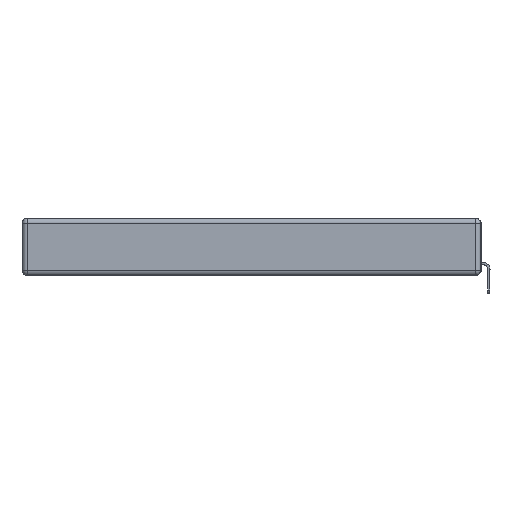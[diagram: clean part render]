
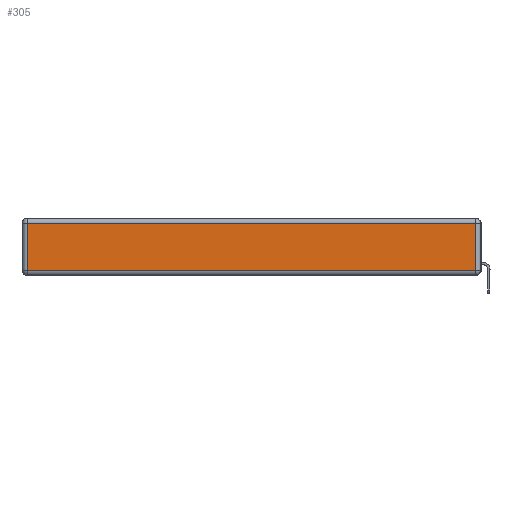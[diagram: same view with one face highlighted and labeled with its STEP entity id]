
A CAD part, left-side view. The second image highlights one B-rep face of the part: STEP entity #305.
In plain terms, the highlighted planar face has unit normal (-1, 0, 0).
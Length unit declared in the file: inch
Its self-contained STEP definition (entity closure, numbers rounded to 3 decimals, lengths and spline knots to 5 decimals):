
#305 = ADVANCED_FACE ( 'NONE', ( #16633 ), #11676, .T. ) ;
#1198 = DIRECTION ( 'NONE',  ( 0., 0., 1. ) ) ;
#1295 = ORIENTED_EDGE ( 'NONE', *, *, #4385, .T. ) ;
#2256 = VERTEX_POINT ( 'NONE', #5201 ) ;
#2484 = ORIENTED_EDGE ( 'NONE', *, *, #16895, .T. ) ;
#2936 = CARTESIAN_POINT ( 'NONE',  ( 0., 0., -0.343 ) ) ;
#4385 = EDGE_CURVE ( 'NONE', #16266, #7479, #18119, .T. ) ;
#4437 = CARTESIAN_POINT ( 'NONE',  ( 0., 2.75, -0.03 ) ) ;
#4552 = LINE ( 'NONE', #4437, #10740 ) ;
#5201 = CARTESIAN_POINT ( 'NONE',  ( 0., 0.03, -0.313 ) ) ;
#6380 = AXIS2_PLACEMENT_3D ( 'NONE', #2936, #9952, #1198 ) ;
#7362 = VERTEX_POINT ( 'NONE', #20991 ) ;
#7479 = VERTEX_POINT ( 'NONE', #11413 ) ;
#8921 = CARTESIAN_POINT ( 'NONE',  ( 0., 2.72, -0.343 ) ) ;
#9952 = DIRECTION ( 'NONE',  ( -1., 0., 0. ) ) ;
#10740 = VECTOR ( 'NONE', #14931, 39.37008 ) ;
#11413 = CARTESIAN_POINT ( 'NONE',  ( 0., 2.72, -0.313 ) ) ;
#11473 = ORIENTED_EDGE ( 'NONE', *, *, #18775, .T. ) ;
#11676 = PLANE ( 'NONE',  #6380 ) ;
#12119 = VECTOR ( 'NONE', #18735, 39.37008 ) ;
#12217 = VECTOR ( 'NONE', #22019, 39.37008 ) ;
#12867 = EDGE_LOOP ( 'NONE', ( #2484, #16663, #11473, #1295 ) ) ;
#13571 = CARTESIAN_POINT ( 'NONE',  ( 0., 0., -0.313 ) ) ;
#14931 = DIRECTION ( 'NONE',  ( 0., 1., 0. ) ) ;
#15064 = LINE ( 'NONE', #13571, #12119 ) ;
#16266 = VERTEX_POINT ( 'NONE', #21402 ) ;
#16633 = FACE_OUTER_BOUND ( 'NONE', #12867, .T. ) ;
#16663 = ORIENTED_EDGE ( 'NONE', *, *, #19182, .T. ) ;
#16895 = EDGE_CURVE ( 'NONE', #7479, #2256, #15064, .T. ) ;
#17077 = CARTESIAN_POINT ( 'NONE',  ( 0., 0.03, -0.343 ) ) ;
#18119 = LINE ( 'NONE', #8921, #21364 ) ;
#18735 = DIRECTION ( 'NONE',  ( 0., -1., 0. ) ) ;
#18775 = EDGE_CURVE ( 'NONE', #7362, #16266, #4552, .T. ) ;
#18794 = LINE ( 'NONE', #17077, #12217 ) ;
#19182 = EDGE_CURVE ( 'NONE', #2256, #7362, #18794, .T. ) ;
#19500 = DIRECTION ( 'NONE',  ( 0., 0., -1. ) ) ;
#20991 = CARTESIAN_POINT ( 'NONE',  ( 0., 0.03, -0.03 ) ) ;
#21364 = VECTOR ( 'NONE', #19500, 39.37008 ) ;
#21402 = CARTESIAN_POINT ( 'NONE',  ( 0., 2.72, -0.03 ) ) ;
#22019 = DIRECTION ( 'NONE',  ( 0., 0., 1. ) ) ;
